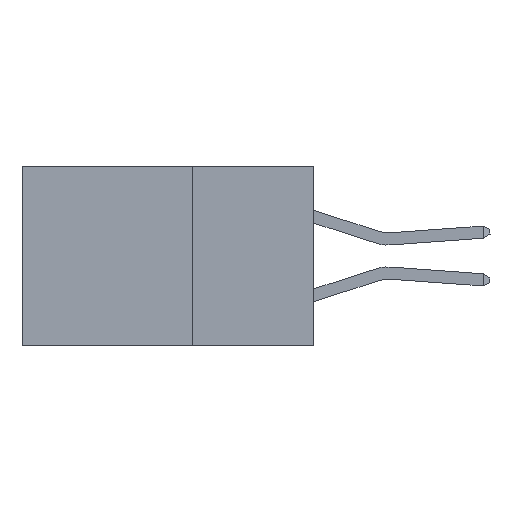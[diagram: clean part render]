
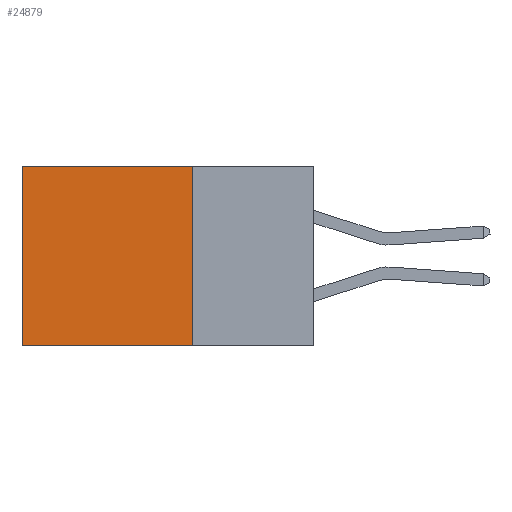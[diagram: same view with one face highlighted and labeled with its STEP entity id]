
A CAD part, left-side view. The second image highlights one B-rep face of the part: STEP entity #24879.
In plain terms, the highlighted planar face has unit normal (-1, 0, 0).
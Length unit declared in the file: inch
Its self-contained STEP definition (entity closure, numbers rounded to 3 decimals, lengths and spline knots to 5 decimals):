
#1382 = VECTOR ( 'NONE', #4414, 39.37008 ) ;
#1499 = LINE ( 'NONE', #35558, #1382 ) ;
#1921 = CARTESIAN_POINT ( 'NONE',  ( 0.2875, 0.25, 0. ) ) ;
#4414 = DIRECTION ( 'NONE',  ( 0., 1., 0. ) ) ;
#4471 = CARTESIAN_POINT ( 'NONE',  ( 0.2875, 0.25, 0. ) ) ;
#4944 = CARTESIAN_POINT ( 'NONE',  ( 0.2875, 0.25, 0. ) ) ;
#5042 = LINE ( 'NONE', #1921, #38316 ) ;
#5330 = ORIENTED_EDGE ( 'NONE', *, *, #19741, .T. ) ;
#6104 = VECTOR ( 'NONE', #10525, 39.37008 ) ;
#8125 = PLANE ( 'NONE',  #16314 ) ;
#10525 = DIRECTION ( 'NONE',  ( 0., 1., 0. ) ) ;
#11254 = DIRECTION ( 'NONE',  ( 0., 0., -1. ) ) ;
#11833 = VERTEX_POINT ( 'NONE', #30369 ) ;
#14595 = DIRECTION ( 'NONE',  ( 1., 0., 0. ) ) ;
#15032 = DIRECTION ( 'NONE',  ( 0., 0., -1. ) ) ;
#15970 = CARTESIAN_POINT ( 'NONE',  ( 0.2875, 0.25, -0.37 ) ) ;
#16314 = AXIS2_PLACEMENT_3D ( 'NONE', #31312, #14595, #11254 ) ;
#18842 = EDGE_CURVE ( 'NONE', #39073, #39945, #1499, .T. ) ;
#19575 = CARTESIAN_POINT ( 'NONE',  ( 0.2875, 0.6, -0.37 ) ) ;
#19741 = EDGE_CURVE ( 'NONE', #25342, #11833, #20337, .T. ) ;
#20337 = LINE ( 'NONE', #4471, #6104 ) ;
#21010 = VECTOR ( 'NONE', #15032, 39.37008 ) ;
#21734 = DIRECTION ( 'NONE',  ( 0., 0., -1. ) ) ;
#24498 = EDGE_CURVE ( 'NONE', #25342, #39073, #5042, .T. ) ;
#24676 = ORIENTED_EDGE ( 'NONE', *, *, #33425, .T. ) ;
#24879 = ADVANCED_FACE ( 'NONE', ( #40730 ), #8125, .F. ) ;
#25342 = VERTEX_POINT ( 'NONE', #4944 ) ;
#26126 = LINE ( 'NONE', #36589, #21010 ) ;
#27423 = ORIENTED_EDGE ( 'NONE', *, *, #18842, .F. ) ;
#28793 = EDGE_LOOP ( 'NONE', ( #24676, #27423, #34081, #5330 ) ) ;
#30369 = CARTESIAN_POINT ( 'NONE',  ( 0.2875, 0.6, 0. ) ) ;
#31312 = CARTESIAN_POINT ( 'NONE',  ( 0.2875, 0.25, 0. ) ) ;
#33425 = EDGE_CURVE ( 'NONE', #11833, #39945, #26126, .T. ) ;
#34081 = ORIENTED_EDGE ( 'NONE', *, *, #24498, .F. ) ;
#35558 = CARTESIAN_POINT ( 'NONE',  ( 0.2875, 0.25, -0.37 ) ) ;
#36589 = CARTESIAN_POINT ( 'NONE',  ( 0.2875, 0.6, 0. ) ) ;
#38316 = VECTOR ( 'NONE', #21734, 39.37008 ) ;
#39073 = VERTEX_POINT ( 'NONE', #15970 ) ;
#39945 = VERTEX_POINT ( 'NONE', #19575 ) ;
#40730 = FACE_OUTER_BOUND ( 'NONE', #28793, .T. ) ;
